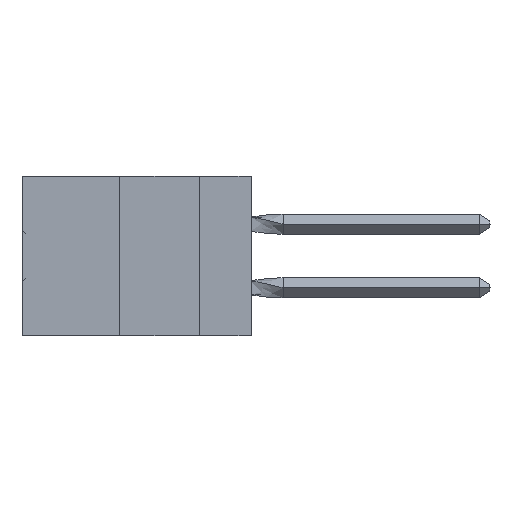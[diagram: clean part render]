
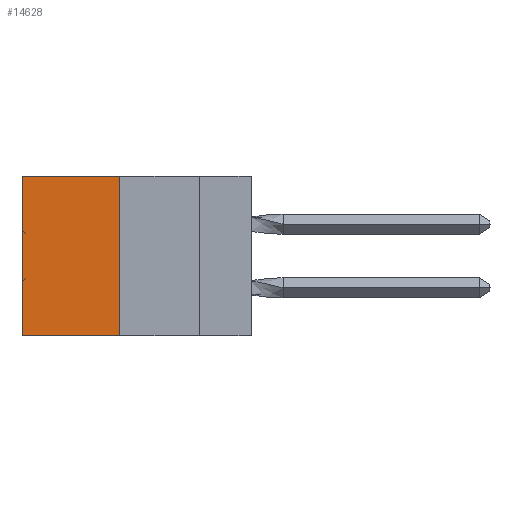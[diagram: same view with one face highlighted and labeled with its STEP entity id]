
A CAD part, left-side view. The second image highlights one B-rep face of the part: STEP entity #14628.
In plain terms, the highlighted planar face has unit normal (-1, 0, 0).
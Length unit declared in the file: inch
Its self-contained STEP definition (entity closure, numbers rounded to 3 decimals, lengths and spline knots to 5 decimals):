
#2236 = DIRECTION ( 'NONE',  ( 1., 0., 0. ) ) ;
#2325 = CARTESIAN_POINT ( 'NONE',  ( 0.305, 0.413, -0.5 ) ) ;
#2992 = CARTESIAN_POINT ( 'NONE',  ( 0.305, 0.413, -0.5 ) ) ;
#3910 = LINE ( 'NONE', #5300, #24910 ) ;
#3965 = VERTEX_POINT ( 'NONE', #41634 ) ;
#5300 = CARTESIAN_POINT ( 'NONE',  ( 0.305, 0.72, -0.5 ) ) ;
#6327 = LINE ( 'NONE', #2992, #16048 ) ;
#7244 = CARTESIAN_POINT ( 'NONE',  ( 0.305, 0.413, -0.5 ) ) ;
#9741 = EDGE_LOOP ( 'NONE', ( #16712, #38626, #32445, #11779 ) ) ;
#11779 = ORIENTED_EDGE ( 'NONE', *, *, #59936, .T. ) ;
#12942 = VECTOR ( 'NONE', #50829, 39.37008 ) ;
#14628 = ADVANCED_FACE ( 'NONE', ( #53986 ), #45506, .F. ) ;
#16048 = VECTOR ( 'NONE', #55724, 39.37008 ) ;
#16627 = VERTEX_POINT ( 'NONE', #24778 ) ;
#16658 = EDGE_CURVE ( 'NONE', #3965, #39626, #46946, .T. ) ;
#16712 = ORIENTED_EDGE ( 'NONE', *, *, #34645, .T. ) ;
#19284 = AXIS2_PLACEMENT_3D ( 'NONE', #7244, #2236, #60340 ) ;
#19939 = DIRECTION ( 'NONE',  ( 0., 0., -1. ) ) ;
#24778 = CARTESIAN_POINT ( 'NONE',  ( 0.305, 0.72, -0.5 ) ) ;
#24910 = VECTOR ( 'NONE', #19939, 39.37008 ) ;
#25498 = VERTEX_POINT ( 'NONE', #57798 ) ;
#32445 = ORIENTED_EDGE ( 'NONE', *, *, #16658, .F. ) ;
#34645 = EDGE_CURVE ( 'NONE', #25498, #16627, #3910, .T. ) ;
#36683 = CARTESIAN_POINT ( 'NONE',  ( 0.305, 0.413, -0.5 ) ) ;
#38626 = ORIENTED_EDGE ( 'NONE', *, *, #54506, .F. ) ;
#39626 = VERTEX_POINT ( 'NONE', #36683 ) ;
#41634 = CARTESIAN_POINT ( 'NONE',  ( 0.305, 0.413, 0. ) ) ;
#44807 = DIRECTION ( 'NONE',  ( 0., 0., -1. ) ) ;
#45506 = PLANE ( 'NONE',  #19284 ) ;
#46946 = LINE ( 'NONE', #2325, #51457 ) ;
#49130 = LINE ( 'NONE', #56251, #12942 ) ;
#50829 = DIRECTION ( 'NONE',  ( 0., 1., 0. ) ) ;
#51457 = VECTOR ( 'NONE', #44807, 39.37008 ) ;
#53986 = FACE_OUTER_BOUND ( 'NONE', #9741, .T. ) ;
#54506 = EDGE_CURVE ( 'NONE', #39626, #16627, #6327, .T. ) ;
#55724 = DIRECTION ( 'NONE',  ( 0., 1., 0. ) ) ;
#56251 = CARTESIAN_POINT ( 'NONE',  ( 0.305, 0.413, 0. ) ) ;
#57798 = CARTESIAN_POINT ( 'NONE',  ( 0.305, 0.72, 0. ) ) ;
#59936 = EDGE_CURVE ( 'NONE', #3965, #25498, #49130, .T. ) ;
#60340 = DIRECTION ( 'NONE',  ( 0., 0., -1. ) ) ;
